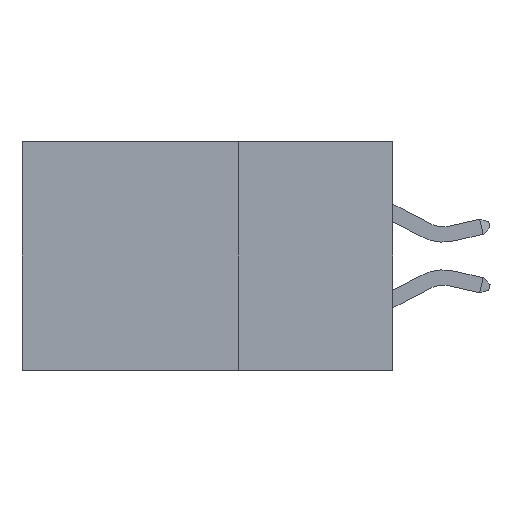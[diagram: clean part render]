
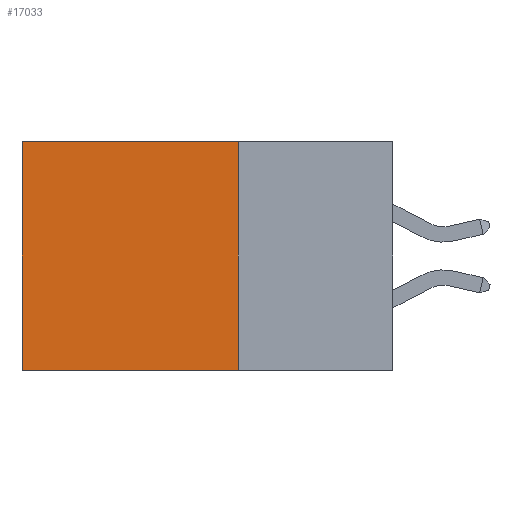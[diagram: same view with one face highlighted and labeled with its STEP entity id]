
A CAD part, left-side view. The second image highlights one B-rep face of the part: STEP entity #17033.
In plain terms, the highlighted planar face has unit normal (-1, 0, 0).
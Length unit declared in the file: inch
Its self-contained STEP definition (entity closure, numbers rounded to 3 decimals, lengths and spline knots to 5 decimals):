
#1300 = PLANE ( 'NONE',  #15717 ) ;
#1363 = DIRECTION ( 'NONE',  ( 0., 0., -1. ) ) ;
#1390 = CARTESIAN_POINT ( 'NONE',  ( 0.2875, 0.25, 0. ) ) ;
#1395 = ORIENTED_EDGE ( 'NONE', *, *, #13267, .F. ) ;
#1515 = VERTEX_POINT ( 'NONE', #1390 ) ;
#1942 = EDGE_CURVE ( 'NONE', #1515, #11940, #3366, .T. ) ;
#2142 = ORIENTED_EDGE ( 'NONE', *, *, #12505, .T. ) ;
#3366 = LINE ( 'NONE', #9034, #20383 ) ;
#4463 = DIRECTION ( 'NONE',  ( 0., 0., -1. ) ) ;
#5762 = LINE ( 'NONE', #10465, #18084 ) ;
#7040 = VERTEX_POINT ( 'NONE', #20267 ) ;
#9034 = CARTESIAN_POINT ( 'NONE',  ( 0.2875, 0.25, 0. ) ) ;
#9125 = DIRECTION ( 'NONE',  ( 0., 1., 0. ) ) ;
#9591 = CARTESIAN_POINT ( 'NONE',  ( 0.2875, 0.6, 0. ) ) ;
#10465 = CARTESIAN_POINT ( 'NONE',  ( 0.2875, 0.25, -0.37 ) ) ;
#11443 = CARTESIAN_POINT ( 'NONE',  ( 0.2875, 0.25, 0. ) ) ;
#11940 = VERTEX_POINT ( 'NONE', #9591 ) ;
#12373 = CARTESIAN_POINT ( 'NONE',  ( 0.2875, 0.25, 0. ) ) ;
#12505 = EDGE_CURVE ( 'NONE', #11940, #7040, #22124, .T. ) ;
#13234 = CARTESIAN_POINT ( 'NONE',  ( 0.2875, 0.25, -0.37 ) ) ;
#13267 = EDGE_CURVE ( 'NONE', #1515, #18212, #24656, .T. ) ;
#13349 = VECTOR ( 'NONE', #4463, 39.37008 ) ;
#14485 = FACE_OUTER_BOUND ( 'NONE', #18191, .T. ) ;
#14543 = EDGE_CURVE ( 'NONE', #18212, #7040, #5762, .T. ) ;
#15410 = DIRECTION ( 'NONE',  ( 1., 0., 0. ) ) ;
#15717 = AXIS2_PLACEMENT_3D ( 'NONE', #11443, #15410, #17796 ) ;
#17033 = ADVANCED_FACE ( 'NONE', ( #14485 ), #1300, .F. ) ;
#17796 = DIRECTION ( 'NONE',  ( 0., 0., -1. ) ) ;
#18084 = VECTOR ( 'NONE', #20519, 39.37008 ) ;
#18132 = ORIENTED_EDGE ( 'NONE', *, *, #1942, .T. ) ;
#18191 = EDGE_LOOP ( 'NONE', ( #2142, #24969, #1395, #18132 ) ) ;
#18212 = VERTEX_POINT ( 'NONE', #13234 ) ;
#19187 = CARTESIAN_POINT ( 'NONE',  ( 0.2875, 0.6, 0. ) ) ;
#20267 = CARTESIAN_POINT ( 'NONE',  ( 0.2875, 0.6, -0.37 ) ) ;
#20383 = VECTOR ( 'NONE', #9125, 39.37008 ) ;
#20519 = DIRECTION ( 'NONE',  ( 0., 1., 0. ) ) ;
#21206 = VECTOR ( 'NONE', #1363, 39.37008 ) ;
#22124 = LINE ( 'NONE', #19187, #21206 ) ;
#24656 = LINE ( 'NONE', #12373, #13349 ) ;
#24969 = ORIENTED_EDGE ( 'NONE', *, *, #14543, .F. ) ;
